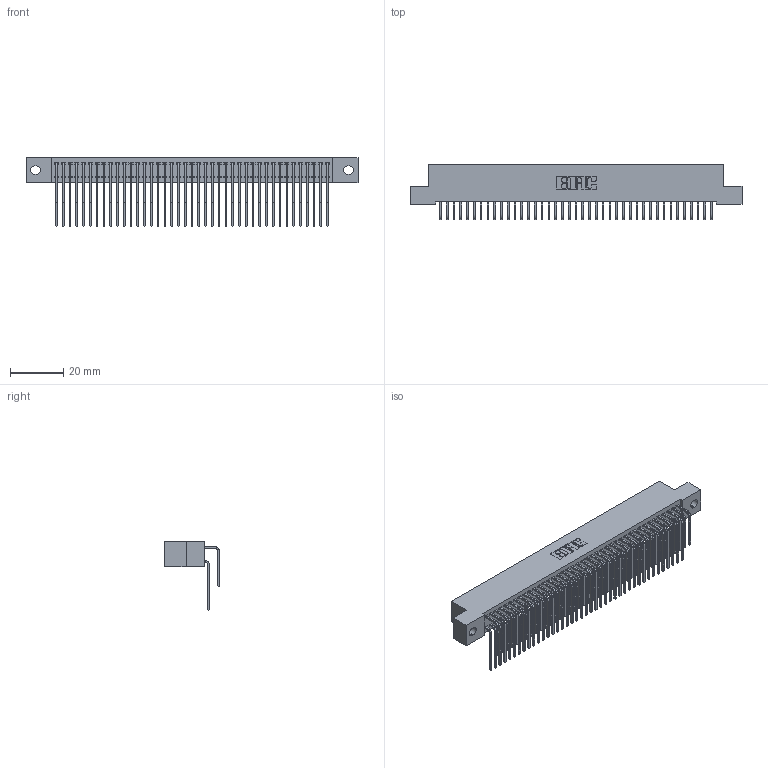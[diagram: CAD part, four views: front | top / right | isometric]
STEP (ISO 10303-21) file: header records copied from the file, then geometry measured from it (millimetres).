
FILE_DESCRIPTION (( 'STEP AP203' ), '1' );
FILE_NAME ('392-082-559-202.STEP', '2018-08-18T04:03:53', ( '' ), ( '' ), 'SwSTEP 2.0', 'SolidWorks 2016', '' );
FILE_SCHEMA (( 'CONFIG_CONTROL_DESIGN' ));
Length unit declared in the file: inch
Products named in the file (4): 345-292-001_558 559 Tail - 1; 345-292-001_559 Tail - 2; 392-082-559-202; 342 Part_.128 Slot
Assembly tree (83 placements, depth 2):
  392-082-559-202
    342 Part_.128 Slot
    345-292-001_558 559 Tail - 1  x41
    345-292-001_559 Tail - 2  x41
Bounding box: 124.46 x 20.64 x 25.78 mm (x, y, z)
Volume: 11598.9 mm3; surface area: 20754.8 mm2
Topology: 83 solids, 83 shells, 4542 faces, 13513 edges, 8898 vertices
Faces by surface type: plane 3186, cylinder 1356
Entity records: 28293 total; most frequent: CARTESIAN_POINT 4741, ORIENTED_EDGE 4626, DIRECTION 4033, EDGE_CURVE 2313, LINE 2145, VECTOR 2145, VERTEX_POINT 1538, AXIS2_PLACEMENT_3D 944
